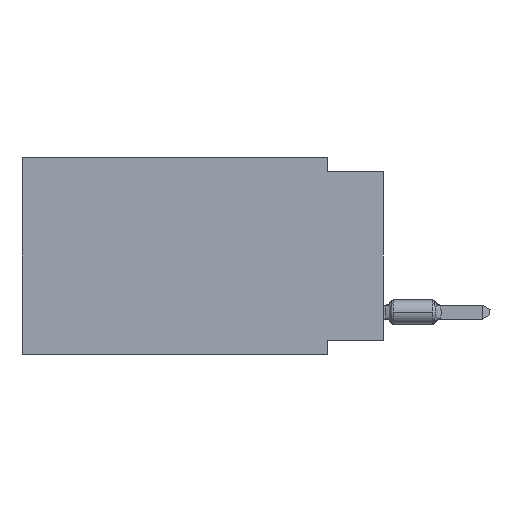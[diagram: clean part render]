
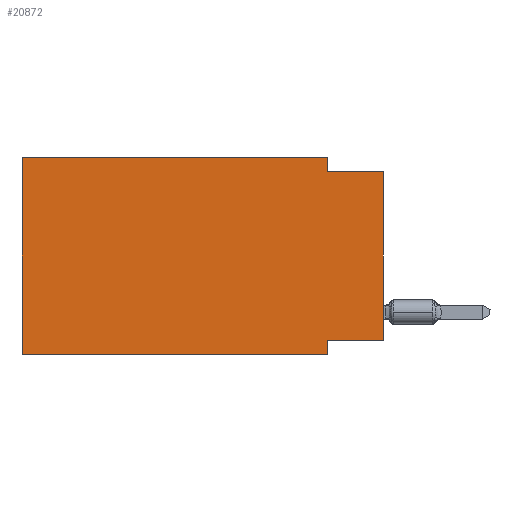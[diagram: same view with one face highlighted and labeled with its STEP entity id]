
A CAD part, left-side view. The second image highlights one B-rep face of the part: STEP entity #20872.
In plain terms, the highlighted planar face has unit normal (-1, 0, 0).
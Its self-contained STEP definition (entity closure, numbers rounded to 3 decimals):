
#444 = EDGE_LOOP ( 'NONE', ( #19641, #18733, #14844, #16732, #2091, #13857, #4167, #4875 ) ) ;
#594 = VERTEX_POINT ( 'NONE', #10977 ) ;
#1433 = VECTOR ( 'NONE', #3708, 1000. ) ;
#1520 = VERTEX_POINT ( 'NONE', #3435 ) ;
#1537 = CARTESIAN_POINT ( 'NONE',  ( 0., 16.383, 0. ) ) ;
#2091 = ORIENTED_EDGE ( 'NONE', *, *, #16657, .F. ) ;
#2573 = VECTOR ( 'NONE', #15178, 1000. ) ;
#3103 = CARTESIAN_POINT ( 'NONE',  ( 0., 16.383, 0. ) ) ;
#3340 = DIRECTION ( 'NONE',  ( 0., 0., 1. ) ) ;
#3435 = CARTESIAN_POINT ( 'NONE',  ( 0., 16.383, -8.89 ) ) ;
#3504 = CARTESIAN_POINT ( 'NONE',  ( 0., 0., -8.255 ) ) ;
#3708 = DIRECTION ( 'NONE',  ( 0., 0., -1. ) ) ;
#3986 = EDGE_CURVE ( 'NONE', #19117, #17978, #14786, .T. ) ;
#4167 = ORIENTED_EDGE ( 'NONE', *, *, #19495, .F. ) ;
#4764 = EDGE_CURVE ( 'NONE', #1520, #23214, #16536, .T. ) ;
#4875 = ORIENTED_EDGE ( 'NONE', *, *, #20469, .F. ) ;
#4912 = CARTESIAN_POINT ( 'NONE',  ( 0., 2.54, 0. ) ) ;
#4926 = DIRECTION ( 'NONE',  ( 0., 0., 1. ) ) ;
#5353 = AXIS2_PLACEMENT_3D ( 'NONE', #3103, #7027, #7138 ) ;
#5530 = VECTOR ( 'NONE', #4926, 1000. ) ;
#5669 = CARTESIAN_POINT ( 'NONE',  ( 0., 2.54, 0. ) ) ;
#6024 = VECTOR ( 'NONE', #9047, 1000. ) ;
#7027 = DIRECTION ( 'NONE',  ( 1., 0., 0. ) ) ;
#7030 = CARTESIAN_POINT ( 'NONE',  ( 0., 0., -8.255 ) ) ;
#7072 = VERTEX_POINT ( 'NONE', #3504 ) ;
#7138 = DIRECTION ( 'NONE',  ( 0., 0., -1. ) ) ;
#7409 = LINE ( 'NONE', #10995, #11823 ) ;
#8111 = EDGE_CURVE ( 'NONE', #594, #19117, #15964, .T. ) ;
#8955 = LINE ( 'NONE', #10567, #16220 ) ;
#9047 = DIRECTION ( 'NONE',  ( 0., -1., 0. ) ) ;
#9763 = EDGE_CURVE ( 'NONE', #7072, #23378, #22128, .T. ) ;
#10567 = CARTESIAN_POINT ( 'NONE',  ( 0., 2.54, -8.89 ) ) ;
#10785 = CARTESIAN_POINT ( 'NONE',  ( 0., 2.54, -8.89 ) ) ;
#10977 = CARTESIAN_POINT ( 'NONE',  ( 0., 16.383, 0. ) ) ;
#10995 = CARTESIAN_POINT ( 'NONE',  ( 0., 0., -0.635 ) ) ;
#11223 = DIRECTION ( 'NONE',  ( 0., 1., 0. ) ) ;
#11239 = DIRECTION ( 'NONE',  ( 0., -1., 0. ) ) ;
#11823 = VECTOR ( 'NONE', #11239, 1000. ) ;
#12193 = CARTESIAN_POINT ( 'NONE',  ( 0., 16.383, 0. ) ) ;
#12714 = CARTESIAN_POINT ( 'NONE',  ( 0., 2.54, -8.255 ) ) ;
#13107 = CARTESIAN_POINT ( 'NONE',  ( 0., 0., -0.635 ) ) ;
#13857 = ORIENTED_EDGE ( 'NONE', *, *, #4764, .T. ) ;
#14786 = LINE ( 'NONE', #5669, #1433 ) ;
#14844 = ORIENTED_EDGE ( 'NONE', *, *, #3986, .F. ) ;
#15178 = DIRECTION ( 'NONE',  ( 0., -1., 0. ) ) ;
#15964 = LINE ( 'NONE', #1537, #6024 ) ;
#16220 = VECTOR ( 'NONE', #23425, 1000. ) ;
#16445 = VERTEX_POINT ( 'NONE', #12714 ) ;
#16471 = EDGE_CURVE ( 'NONE', #17978, #23378, #7409, .T. ) ;
#16503 = LINE ( 'NONE', #7030, #19902 ) ;
#16536 = LINE ( 'NONE', #20328, #2573 ) ;
#16657 = EDGE_CURVE ( 'NONE', #1520, #594, #17602, .T. ) ;
#16710 = CARTESIAN_POINT ( 'NONE',  ( 0., 2.54, -0.635 ) ) ;
#16732 = ORIENTED_EDGE ( 'NONE', *, *, #8111, .F. ) ;
#17602 = LINE ( 'NONE', #12193, #5530 ) ;
#17978 = VERTEX_POINT ( 'NONE', #16710 ) ;
#18576 = FACE_OUTER_BOUND ( 'NONE', #444, .T. ) ;
#18733 = ORIENTED_EDGE ( 'NONE', *, *, #16471, .F. ) ;
#19117 = VERTEX_POINT ( 'NONE', #4912 ) ;
#19495 = EDGE_CURVE ( 'NONE', #16445, #23214, #8955, .T. ) ;
#19641 = ORIENTED_EDGE ( 'NONE', *, *, #9763, .T. ) ;
#19902 = VECTOR ( 'NONE', #11223, 1000. ) ;
#20328 = CARTESIAN_POINT ( 'NONE',  ( 0., 16.383, -8.89 ) ) ;
#20469 = EDGE_CURVE ( 'NONE', #7072, #16445, #16503, .T. ) ;
#20872 = ADVANCED_FACE ( 'NONE', ( #18576 ), #23849, .F. ) ;
#22128 = LINE ( 'NONE', #22372, #24009 ) ;
#22372 = CARTESIAN_POINT ( 'NONE',  ( 0., 0., 0. ) ) ;
#23214 = VERTEX_POINT ( 'NONE', #10785 ) ;
#23378 = VERTEX_POINT ( 'NONE', #13107 ) ;
#23425 = DIRECTION ( 'NONE',  ( 0., 0., -1. ) ) ;
#23849 = PLANE ( 'NONE',  #5353 ) ;
#24009 = VECTOR ( 'NONE', #3340, 1000. ) ;
